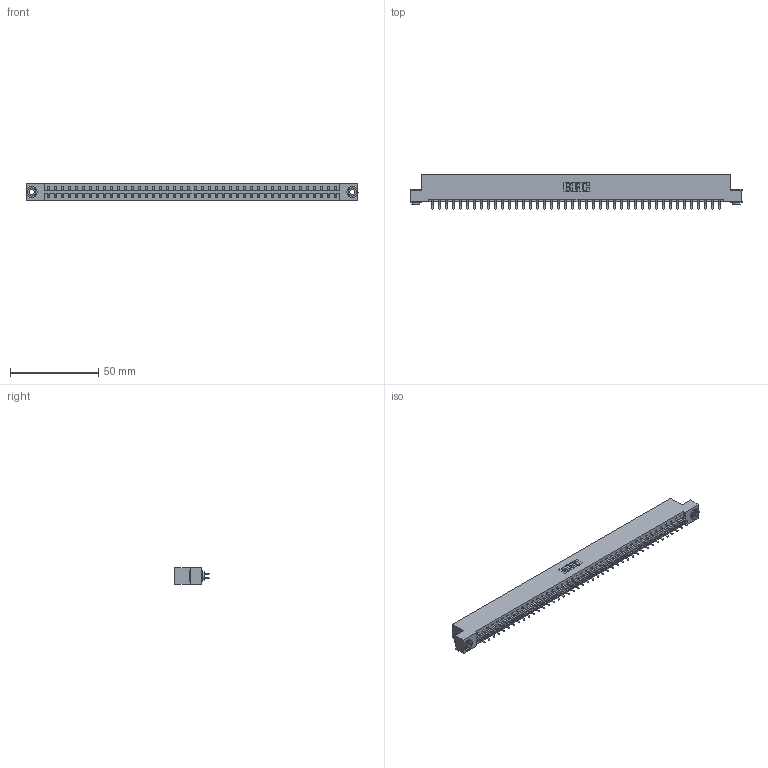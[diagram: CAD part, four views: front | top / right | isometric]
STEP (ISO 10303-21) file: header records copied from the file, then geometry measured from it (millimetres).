
FILE_DESCRIPTION (( 'STEP AP203' ), '1' );
FILE_NAME ('333-084-556-203.STEP', '2018-08-05T05:03:10', ( '' ), ( '' ), 'SwSTEP 2.0', 'SolidWorks 2016', '' );
FILE_SCHEMA (( 'CONFIG_CONTROL_DESIGN' ));
Length unit declared in the file: inch
Products named in the file (4): 345-292-001_556 Tail; 345-250-002_345-250-002-102; 333-084-556-203; 333 Part_Flush - .156 Dia - TH
Assembly tree (87 placements, depth 2):
  333-084-556-203
    333 Part_Flush - .156 Dia - TH
    345-292-001_556 Tail  x84
    345-250-002_345-250-002-102  x2
Bounding box: 187.96 x 19.57 x 9.4 mm (x, y, z)
Volume: 19205.7 mm3; surface area: 22844 mm2
Topology: 87 solids, 87 shells, 5024 faces, 14919 edges, 9830 vertices
Faces by surface type: plane 3440, cylinder 1576, cone 8
Entity records: 27890 total; most frequent: CARTESIAN_POINT 4613, ORIENTED_EDGE 4530, DIRECTION 3963, EDGE_CURVE 2265, VECTOR 2105, LINE 2105, VERTEX_POINT 1506, AXIS2_PLACEMENT_3D 929
